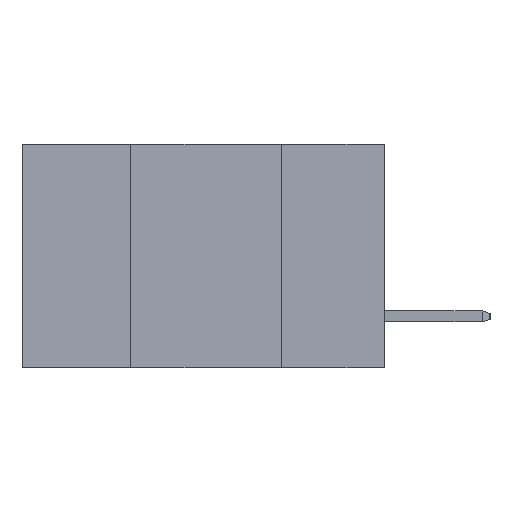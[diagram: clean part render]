
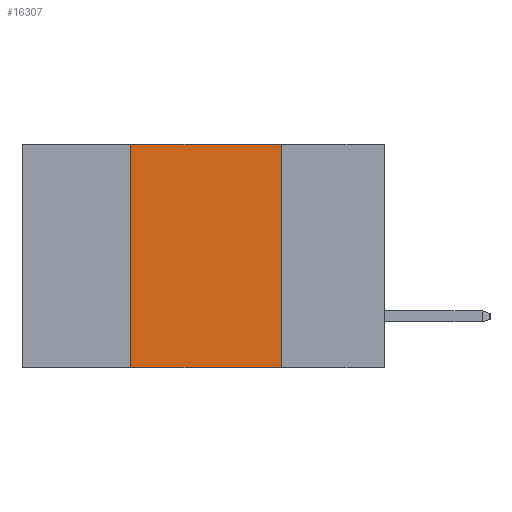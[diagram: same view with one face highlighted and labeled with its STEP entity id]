
A CAD part, left-side view. The second image highlights one B-rep face of the part: STEP entity #16307.
In plain terms, the highlighted planar face has unit normal (-1, 0, 0).
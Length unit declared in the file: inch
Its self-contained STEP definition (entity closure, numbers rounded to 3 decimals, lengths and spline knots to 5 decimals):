
#227 = CARTESIAN_POINT ( 'NONE',  ( 0., 0.6, 0. ) ) ;
#297 = PLANE ( 'NONE',  #17748 ) ;
#654 = VECTOR ( 'NONE', #6348, 39.37008 ) ;
#1625 = VERTEX_POINT ( 'NONE', #4622 ) ;
#2125 = LINE ( 'NONE', #9576, #18788 ) ;
#2490 = EDGE_CURVE ( 'NONE', #18516, #1625, #13007, .T. ) ;
#2648 = ORIENTED_EDGE ( 'NONE', *, *, #16815, .F. ) ;
#2649 = EDGE_CURVE ( 'NONE', #14832, #12384, #6074, .T. ) ;
#2981 = EDGE_LOOP ( 'NONE', ( #9924, #5866, #2648, #10901 ) ) ;
#3471 = LINE ( 'NONE', #9636, #19171 ) ;
#4098 = FACE_OUTER_BOUND ( 'NONE', #2981, .T. ) ;
#4622 = CARTESIAN_POINT ( 'NONE',  ( 0., 0.17, -0.37 ) ) ;
#4981 = EDGE_CURVE ( 'NONE', #12384, #1625, #3471, .T. ) ;
#5079 = DIRECTION ( 'NONE',  ( 0., 0., -1. ) ) ;
#5394 = DIRECTION ( 'NONE',  ( 0., -1., 0. ) ) ;
#5866 = ORIENTED_EDGE ( 'NONE', *, *, #2649, .F. ) ;
#6074 = LINE ( 'NONE', #8579, #17641 ) ;
#6335 = CARTESIAN_POINT ( 'NONE',  ( 0., 0.17, 0. ) ) ;
#6348 = DIRECTION ( 'NONE',  ( 0., -1., 0. ) ) ;
#8579 = CARTESIAN_POINT ( 'NONE',  ( 0., 0.6, 0. ) ) ;
#9576 = CARTESIAN_POINT ( 'NONE',  ( 0., 0.42, 0. ) ) ;
#9636 = CARTESIAN_POINT ( 'NONE',  ( 0., 0.17, 0. ) ) ;
#9924 = ORIENTED_EDGE ( 'NONE', *, *, #4981, .F. ) ;
#10722 = DIRECTION ( 'NONE',  ( 0., 0., -1. ) ) ;
#10837 = CARTESIAN_POINT ( 'NONE',  ( 0., 0.6, -0.37 ) ) ;
#10901 = ORIENTED_EDGE ( 'NONE', *, *, #2490, .T. ) ;
#11055 = DIRECTION ( 'NONE',  ( 0., 0., 1. ) ) ;
#12384 = VERTEX_POINT ( 'NONE', #6335 ) ;
#13007 = LINE ( 'NONE', #10837, #654 ) ;
#14219 = DIRECTION ( 'NONE',  ( 1., 0., 0. ) ) ;
#14832 = VERTEX_POINT ( 'NONE', #16034 ) ;
#15194 = CARTESIAN_POINT ( 'NONE',  ( 0., 0.42, -0.37 ) ) ;
#16034 = CARTESIAN_POINT ( 'NONE',  ( 0., 0.42, 0. ) ) ;
#16307 = ADVANCED_FACE ( 'NONE', ( #4098 ), #297, .F. ) ;
#16815 = EDGE_CURVE ( 'NONE', #18516, #14832, #2125, .T. ) ;
#17641 = VECTOR ( 'NONE', #5394, 39.37008 ) ;
#17748 = AXIS2_PLACEMENT_3D ( 'NONE', #227, #14219, #5079 ) ;
#18516 = VERTEX_POINT ( 'NONE', #15194 ) ;
#18788 = VECTOR ( 'NONE', #11055, 39.37008 ) ;
#19171 = VECTOR ( 'NONE', #10722, 39.37008 ) ;
